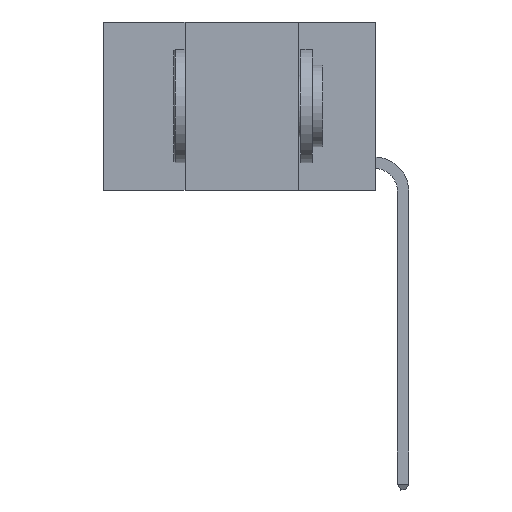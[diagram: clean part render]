
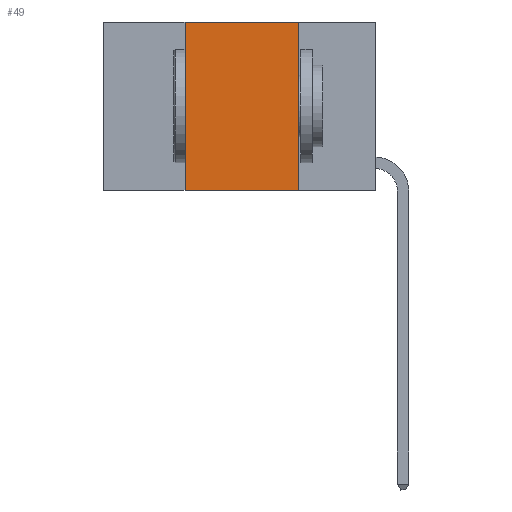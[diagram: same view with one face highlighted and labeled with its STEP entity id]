
A CAD part, left-side view. The second image highlights one B-rep face of the part: STEP entity #49.
In plain terms, the highlighted planar face has unit normal (-1, 0, 0).
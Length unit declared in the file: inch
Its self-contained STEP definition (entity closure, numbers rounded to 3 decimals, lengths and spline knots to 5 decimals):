
#49 = ADVANCED_FACE ( 'NONE', ( #7920 ), #6282, .F. ) ;
#116 = CARTESIAN_POINT ( 'NONE',  ( 0., 0.6, -0.37 ) ) ;
#291 = CARTESIAN_POINT ( 'NONE',  ( 0., 0.42, 0. ) ) ;
#432 = CARTESIAN_POINT ( 'NONE',  ( 0., 0.42, -0.37 ) ) ;
#599 = VECTOR ( 'NONE', #3441, 39.37008 ) ;
#613 = LINE ( 'NONE', #3994, #8733 ) ;
#696 = DIRECTION ( 'NONE',  ( 1., 0., 0. ) ) ;
#1115 = CARTESIAN_POINT ( 'NONE',  ( 0., 0.42, 0. ) ) ;
#1565 = CARTESIAN_POINT ( 'NONE',  ( 0., 0.6, 0. ) ) ;
#2383 = VECTOR ( 'NONE', #2808, 39.37008 ) ;
#2577 = LINE ( 'NONE', #10390, #10379 ) ;
#2743 = VERTEX_POINT ( 'NONE', #432 ) ;
#2808 = DIRECTION ( 'NONE',  ( 0., 0., 1. ) ) ;
#2964 = DIRECTION ( 'NONE',  ( 0., 0., -1. ) ) ;
#3112 = EDGE_CURVE ( 'NONE', #2743, #3344, #7949, .T. ) ;
#3344 = VERTEX_POINT ( 'NONE', #291 ) ;
#3441 = DIRECTION ( 'NONE',  ( 0., -1., 0. ) ) ;
#3915 = CARTESIAN_POINT ( 'NONE',  ( 0., 0.17, 0. ) ) ;
#3982 = ORIENTED_EDGE ( 'NONE', *, *, #4512, .T. ) ;
#3994 = CARTESIAN_POINT ( 'NONE',  ( 0., 0.6, 0. ) ) ;
#4255 = LINE ( 'NONE', #116, #599 ) ;
#4298 = VERTEX_POINT ( 'NONE', #7874 ) ;
#4512 = EDGE_CURVE ( 'NONE', #2743, #4298, #4255, .T. ) ;
#4930 = EDGE_LOOP ( 'NONE', ( #9107, #5509, #5556, #3982 ) ) ;
#5203 = VERTEX_POINT ( 'NONE', #3915 ) ;
#5509 = ORIENTED_EDGE ( 'NONE', *, *, #7947, .F. ) ;
#5556 = ORIENTED_EDGE ( 'NONE', *, *, #3112, .F. ) ;
#5579 = EDGE_CURVE ( 'NONE', #5203, #4298, #2577, .T. ) ;
#6282 = PLANE ( 'NONE',  #8573 ) ;
#7384 = DIRECTION ( 'NONE',  ( 0., 0., -1. ) ) ;
#7874 = CARTESIAN_POINT ( 'NONE',  ( 0., 0.17, -0.37 ) ) ;
#7920 = FACE_OUTER_BOUND ( 'NONE', #4930, .T. ) ;
#7947 = EDGE_CURVE ( 'NONE', #3344, #5203, #613, .T. ) ;
#7949 = LINE ( 'NONE', #1115, #2383 ) ;
#8573 = AXIS2_PLACEMENT_3D ( 'NONE', #1565, #696, #7384 ) ;
#8733 = VECTOR ( 'NONE', #10661, 39.37008 ) ;
#9107 = ORIENTED_EDGE ( 'NONE', *, *, #5579, .F. ) ;
#10379 = VECTOR ( 'NONE', #2964, 39.37008 ) ;
#10390 = CARTESIAN_POINT ( 'NONE',  ( 0., 0.17, 0. ) ) ;
#10661 = DIRECTION ( 'NONE',  ( 0., -1., 0. ) ) ;
